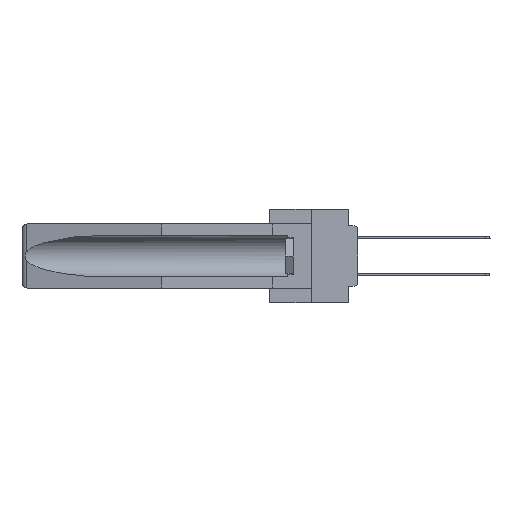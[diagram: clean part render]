
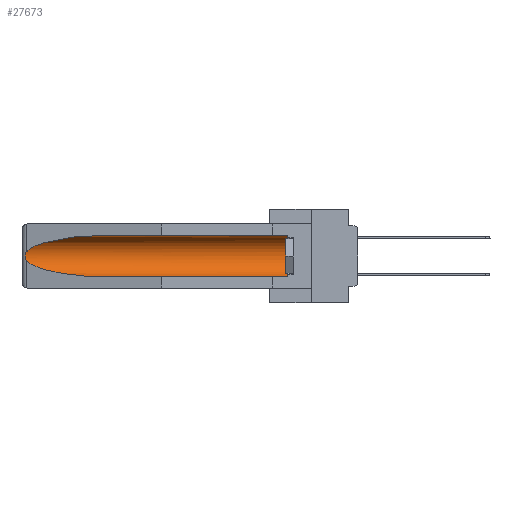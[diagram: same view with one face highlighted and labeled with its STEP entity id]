
A CAD part, left-side view. The second image highlights one B-rep face of the part: STEP entity #27673.
In plain terms, the highlighted cylindrical face has radius 2.857 mm (diameter 5.715 mm), a partial arc.
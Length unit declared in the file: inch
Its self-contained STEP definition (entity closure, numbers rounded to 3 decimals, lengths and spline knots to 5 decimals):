
#12 = LINE ( 'NONE', #20324, #27548 ) ;
#242 = CARTESIAN_POINT ( 'NONE',  ( 0.21114, 1.30732, -0.284 ) ) ;
#655 = EDGE_CURVE ( 'NONE', #29293, #24911, #30964, .T. ) ;
#732 = CARTESIAN_POINT ( 'NONE',  ( 0.21114, 1.30732, -0.059 ) ) ;
#1106 = CARTESIAN_POINT ( 'NONE',  ( 0.26654, 1.53092, -0.15636 ) ) ;
#1436 = CARTESIAN_POINT ( 'NONE',  ( 0.155, 1.07973, -0.284 ) ) ;
#1952 = ORIENTED_EDGE ( 'NONE', *, *, #13672, .T. ) ;
#2754 = CIRCLE ( 'NONE', #25638, 0.1125 ) ;
#2950 = DIRECTION ( 'NONE',  ( 0., -1., 0. ) ) ;
#3368 = VERTEX_POINT ( 'NONE', #18979 ) ;
#5491 = ORIENTED_EDGE ( 'NONE', *, *, #655, .F. ) ;
#5892 = CARTESIAN_POINT ( 'NONE',  ( 0.25451, 1.48313, -0.09465 ) ) ;
#6103 = CARTESIAN_POINT ( 'NONE',  ( 0.2675, 1.53308, -0.17534 ) ) ;
#7730 = ORIENTED_EDGE ( 'NONE', *, *, #28845, .T. ) ;
#8399 = CARTESIAN_POINT ( 'NONE',  ( 0.26537, 1.52718, -0.14972 ) ) ;
#8891 = CYLINDRICAL_SURFACE ( 'NONE', #30561, 0.1125 ) ;
#9223 = DIRECTION ( 'NONE',  ( 0., 0., 1. ) ) ;
#10254 = CARTESIAN_POINT ( 'NONE',  ( 0.155, 1.07973, -0.284 ) ) ;
#11495 =( BOUNDED_CURVE ( )  B_SPLINE_CURVE ( 3, ( #15264, #20241, #242, #10254 ),
 .UNSPECIFIED., .F., .F. ) 
 B_SPLINE_CURVE_WITH_KNOTS ( ( 4, 4 ),
 ( 0.1948, 1.5708 ),
 .UNSPECIFIED. ) 
 CURVE ( )  GEOMETRIC_REPRESENTATION_ITEM ( )  RATIONAL_B_SPLINE_CURVE ( ( 1., 0.848, 0.848, 1. ) ) 
 REPRESENTATION_ITEM ( '' )  );
#11942 = CARTESIAN_POINT ( 'NONE',  ( 0.26655, 1.53094, -0.18657 ) ) ;
#13327 = ORIENTED_EDGE ( 'NONE', *, *, #32521, .T. ) ;
#13620 = CARTESIAN_POINT ( 'NONE',  ( 0.26537, 1.52718, -0.14972 ) ) ;
#13672 = EDGE_CURVE ( 'NONE', #30813, #3368, #12, .T. ) ;
#14114 = CARTESIAN_POINT ( 'NONE',  ( 0.26537, 1.52718, -0.19328 ) ) ;
#15264 = CARTESIAN_POINT ( 'NONE',  ( 0.26537, 1.52718, -0.19328 ) ) ;
#15882 = VECTOR ( 'NONE', #23138, 39.37008 ) ;
#16738 = DIRECTION ( 'NONE',  ( 0., 1., 0. ) ) ;
#18476 = EDGE_CURVE ( 'NONE', #19364, #24911, #11495, .T. ) ;
#18979 = CARTESIAN_POINT ( 'NONE',  ( 0.155, 1.07973, -0.059 ) ) ;
#19364 = VERTEX_POINT ( 'NONE', #30275 ) ;
#19406 = EDGE_CURVE ( 'NONE', #29293, #30813, #2754, .T. ) ;
#20241 = CARTESIAN_POINT ( 'NONE',  ( 0.25451, 1.48313, -0.24835 ) ) ;
#20303 = ORIENTED_EDGE ( 'NONE', *, *, #18476, .T. ) ;
#20324 = CARTESIAN_POINT ( 'NONE',  ( 0.155, -0.30754, -0.059 ) ) ;
#20443 = DIRECTION ( 'NONE',  ( 0., 0., 1. ) ) ;
#21257 = CARTESIAN_POINT ( 'NONE',  ( 0.26597, 1.52961, -0.15275 ) ) ;
#21611 = CARTESIAN_POINT ( 'NONE',  ( 0.155, 0.126, -0.059 ) ) ;
#21775 = VERTEX_POINT ( 'NONE', #25979 ) ;
#23138 = DIRECTION ( 'NONE',  ( 0., 1., 0. ) ) ;
#23304 = CARTESIAN_POINT ( 'NONE',  ( 0.155, -0.30754, -0.284 ) ) ;
#23469 = B_SPLINE_CURVE_WITH_KNOTS ( 'NONE', 3,
 ( #13620, #21257, #1106, #31575, #31416, #6103, #29094, #11942, #24754, #14114 ),
 .UNSPECIFIED., .F., .F.,
 ( 4, 2, 2, 2, 4 ),
 ( 0., 0.00029, 0.00058, 0.00087, 0.00117 ),
 .UNSPECIFIED. ) ;
#24042 = FACE_OUTER_BOUND ( 'NONE', #27935, .T. ) ;
#24696 = CARTESIAN_POINT ( 'NONE',  ( 0.155, -0.30754, -0.1715 ) ) ;
#24754 = CARTESIAN_POINT ( 'NONE',  ( 0.26597, 1.5296, -0.19026 ) ) ;
#24911 = VERTEX_POINT ( 'NONE', #1436 ) ;
#25638 = AXIS2_PLACEMENT_3D ( 'NONE', #30437, #2950, #20443 ) ;
#25979 = CARTESIAN_POINT ( 'NONE',  ( 0.26537, 1.52718, -0.14972 ) ) ;
#27548 = VECTOR ( 'NONE', #30483, 39.37008 ) ;
#27673 = ADVANCED_FACE ( 'NONE', ( #24042 ), #8891, .F. ) ;
#27935 = EDGE_LOOP ( 'NONE', ( #7730, #13327, #20303, #5491, #31496, #1952 ) ) ;
#28505 = CARTESIAN_POINT ( 'NONE',  ( 0.155, 0.126, -0.284 ) ) ;
#28543 = CARTESIAN_POINT ( 'NONE',  ( 0.155, 1.07973, -0.059 ) ) ;
#28845 = EDGE_CURVE ( 'NONE', #3368, #21775, #32359, .T. ) ;
#29094 = CARTESIAN_POINT ( 'NONE',  ( 0.2673, 1.53269, -0.17917 ) ) ;
#29293 = VERTEX_POINT ( 'NONE', #28505 ) ;
#30275 = CARTESIAN_POINT ( 'NONE',  ( 0.26537, 1.52718, -0.19328 ) ) ;
#30437 = CARTESIAN_POINT ( 'NONE',  ( 0.155, 0.126, -0.1715 ) ) ;
#30483 = DIRECTION ( 'NONE',  ( 0., 1., 0. ) ) ;
#30561 = AXIS2_PLACEMENT_3D ( 'NONE', #24696, #16738, #9223 ) ;
#30813 = VERTEX_POINT ( 'NONE', #21611 ) ;
#30964 = LINE ( 'NONE', #23304, #15882 ) ;
#31416 = CARTESIAN_POINT ( 'NONE',  ( 0.2675, 1.53308, -0.16763 ) ) ;
#31496 = ORIENTED_EDGE ( 'NONE', *, *, #19406, .T. ) ;
#31575 = CARTESIAN_POINT ( 'NONE',  ( 0.2673, 1.5327, -0.16383 ) ) ;
#32359 =( BOUNDED_CURVE ( )  B_SPLINE_CURVE ( 3, ( #28543, #732, #5892, #8399 ),
 .UNSPECIFIED., .F., .F. ) 
 B_SPLINE_CURVE_WITH_KNOTS ( ( 4, 4 ),
 ( 4.71239, 6.08839 ),
 .UNSPECIFIED. ) 
 CURVE ( )  GEOMETRIC_REPRESENTATION_ITEM ( )  RATIONAL_B_SPLINE_CURVE ( ( 1., 0.848, 0.848, 1. ) ) 
 REPRESENTATION_ITEM ( '' )  );
#32521 = EDGE_CURVE ( 'NONE', #21775, #19364, #23469, .T. ) ;
